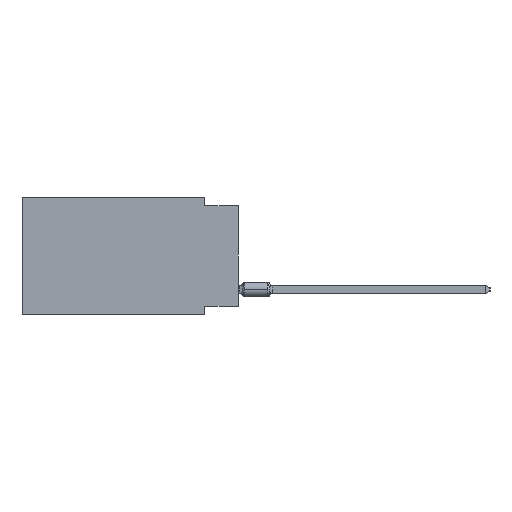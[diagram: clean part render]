
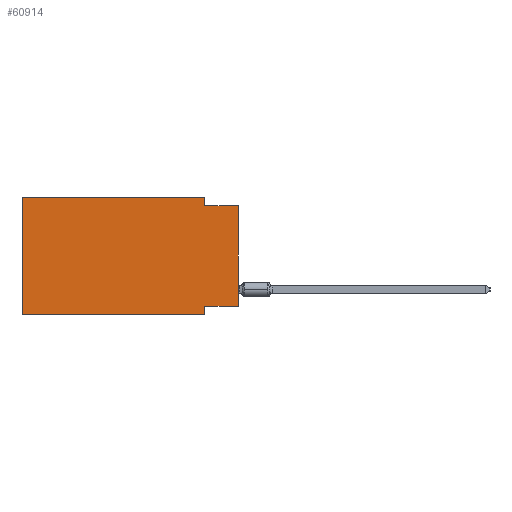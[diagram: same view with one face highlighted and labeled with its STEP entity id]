
A CAD part, left-side view. The second image highlights one B-rep face of the part: STEP entity #60914.
In plain terms, the highlighted planar face has unit normal (-1, 0, 0).
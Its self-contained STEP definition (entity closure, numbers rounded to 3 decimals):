
#1174 = CARTESIAN_POINT ( 'NONE',  ( 0., 2.54, -0.635 ) ) ;
#2150 = CARTESIAN_POINT ( 'NONE',  ( 0., 2.54, 0. ) ) ;
#3774 = VERTEX_POINT ( 'NONE', #1174 ) ;
#4014 = LINE ( 'NONE', #15110, #17051 ) ;
#4337 = EDGE_CURVE ( 'NONE', #35056, #33675, #51425, .T. ) ;
#5012 = LINE ( 'NONE', #29210, #55380 ) ;
#9672 = ORIENTED_EDGE ( 'NONE', *, *, #60239, .T. ) ;
#13193 = CARTESIAN_POINT ( 'NONE',  ( 0., 0., -0.635 ) ) ;
#13254 = LINE ( 'NONE', #2150, #56403 ) ;
#14714 = DIRECTION ( 'NONE',  ( 0., 1., 0. ) ) ;
#15110 = CARTESIAN_POINT ( 'NONE',  ( 0., 0., -8.255 ) ) ;
#17051 = VECTOR ( 'NONE', #14714, 1000. ) ;
#19155 = DIRECTION ( 'NONE',  ( 0., -1., 0. ) ) ;
#21648 = LINE ( 'NONE', #45854, #44499 ) ;
#22668 = EDGE_CURVE ( 'NONE', #77616, #57221, #39429, .T. ) ;
#24308 = VERTEX_POINT ( 'NONE', #63778 ) ;
#24437 = VECTOR ( 'NONE', #19155, 1000. ) ;
#25458 = ORIENTED_EDGE ( 'NONE', *, *, #22668, .F. ) ;
#27891 = EDGE_CURVE ( 'NONE', #33675, #24308, #21648, .T. ) ;
#28768 = VECTOR ( 'NONE', #65189, 1000. ) ;
#29210 = CARTESIAN_POINT ( 'NONE',  ( 0., 0., -0.635 ) ) ;
#31074 = EDGE_CURVE ( 'NONE', #37340, #77616, #4014, .T. ) ;
#31951 = ORIENTED_EDGE ( 'NONE', *, *, #36353, .F. ) ;
#33031 = CARTESIAN_POINT ( 'NONE',  ( 0., 2.54, -8.89 ) ) ;
#33675 = VERTEX_POINT ( 'NONE', #70813 ) ;
#33956 = DIRECTION ( 'NONE',  ( 0., -1., 0. ) ) ;
#35056 = VERTEX_POINT ( 'NONE', #59689 ) ;
#35163 = AXIS2_PLACEMENT_3D ( 'NONE', #39660, #58291, #40052 ) ;
#36353 = EDGE_CURVE ( 'NONE', #3774, #72721, #5012, .T. ) ;
#37340 = VERTEX_POINT ( 'NONE', #61921 ) ;
#39138 = DIRECTION ( 'NONE',  ( 0., 0., 1. ) ) ;
#39429 = LINE ( 'NONE', #63606, #40378 ) ;
#39660 = CARTESIAN_POINT ( 'NONE',  ( 0., 16.383, 0. ) ) ;
#40052 = DIRECTION ( 'NONE',  ( 0., 0., -1. ) ) ;
#40378 = VECTOR ( 'NONE', #62431, 1000. ) ;
#42191 = CARTESIAN_POINT ( 'NONE',  ( 0., 0., 0. ) ) ;
#43051 = DIRECTION ( 'NONE',  ( 0., 0., -1. ) ) ;
#44499 = VECTOR ( 'NONE', #33956, 1000. ) ;
#45854 = CARTESIAN_POINT ( 'NONE',  ( 0., 16.383, 0. ) ) ;
#46012 = FACE_OUTER_BOUND ( 'NONE', #65001, .T. ) ;
#48524 = LINE ( 'NONE', #42191, #28768 ) ;
#48970 = VECTOR ( 'NONE', #39138, 1000. ) ;
#51172 = EDGE_CURVE ( 'NONE', #35056, #57221, #73897, .T. ) ;
#51425 = LINE ( 'NONE', #69260, #48970 ) ;
#53433 = DIRECTION ( 'NONE',  ( 0., -1., 0. ) ) ;
#55380 = VECTOR ( 'NONE', #53433, 1000. ) ;
#55659 = CARTESIAN_POINT ( 'NONE',  ( 0., 16.383, -8.89 ) ) ;
#55891 = ORIENTED_EDGE ( 'NONE', *, *, #27891, .F. ) ;
#56403 = VECTOR ( 'NONE', #43051, 1000. ) ;
#57221 = VERTEX_POINT ( 'NONE', #33031 ) ;
#57408 = ORIENTED_EDGE ( 'NONE', *, *, #4337, .F. ) ;
#58291 = DIRECTION ( 'NONE',  ( 1., 0., 0. ) ) ;
#58762 = EDGE_CURVE ( 'NONE', #24308, #3774, #13254, .T. ) ;
#59689 = CARTESIAN_POINT ( 'NONE',  ( 0., 16.383, -8.89 ) ) ;
#60239 = EDGE_CURVE ( 'NONE', #37340, #72721, #48524, .T. ) ;
#60914 = ADVANCED_FACE ( 'NONE', ( #46012 ), #69790, .F. ) ;
#61921 = CARTESIAN_POINT ( 'NONE',  ( 0., 0., -8.255 ) ) ;
#61938 = ORIENTED_EDGE ( 'NONE', *, *, #51172, .T. ) ;
#62431 = DIRECTION ( 'NONE',  ( 0., 0., -1. ) ) ;
#63606 = CARTESIAN_POINT ( 'NONE',  ( 0., 2.54, -8.89 ) ) ;
#63778 = CARTESIAN_POINT ( 'NONE',  ( 0., 2.54, 0. ) ) ;
#65001 = EDGE_LOOP ( 'NONE', ( #9672, #31951, #72394, #55891, #57408, #61938, #25458, #65294 ) ) ;
#65189 = DIRECTION ( 'NONE',  ( 0., 0., 1. ) ) ;
#65294 = ORIENTED_EDGE ( 'NONE', *, *, #31074, .F. ) ;
#69260 = CARTESIAN_POINT ( 'NONE',  ( 0., 16.383, 0. ) ) ;
#69790 = PLANE ( 'NONE',  #35163 ) ;
#70813 = CARTESIAN_POINT ( 'NONE',  ( 0., 16.383, 0. ) ) ;
#71754 = CARTESIAN_POINT ( 'NONE',  ( 0., 2.54, -8.255 ) ) ;
#72394 = ORIENTED_EDGE ( 'NONE', *, *, #58762, .F. ) ;
#72721 = VERTEX_POINT ( 'NONE', #13193 ) ;
#73897 = LINE ( 'NONE', #55659, #24437 ) ;
#77616 = VERTEX_POINT ( 'NONE', #71754 ) ;
